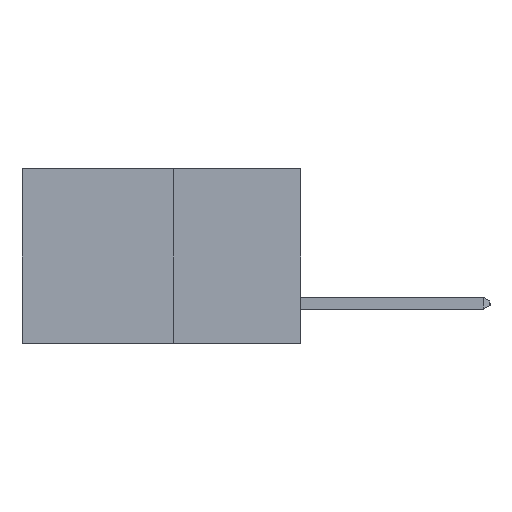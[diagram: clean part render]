
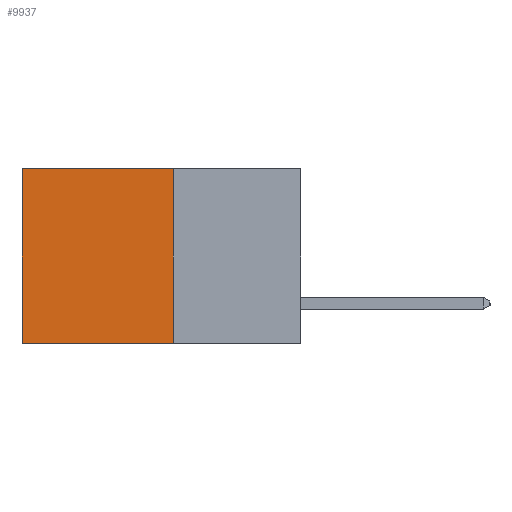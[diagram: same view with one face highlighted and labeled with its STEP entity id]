
A CAD part, left-side view. The second image highlights one B-rep face of the part: STEP entity #9937.
In plain terms, the highlighted planar face has unit normal (-1, 0, 0).
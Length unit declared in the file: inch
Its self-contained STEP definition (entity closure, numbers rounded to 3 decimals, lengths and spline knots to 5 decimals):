
#439 = EDGE_CURVE ( 'NONE', #6047, #4865, #7994, .T. ) ;
#1442 = FACE_OUTER_BOUND ( 'NONE', #7713, .T. ) ;
#1578 = LINE ( 'NONE', #4996, #12822 ) ;
#1787 = DIRECTION ( 'NONE',  ( 0., 1., 0. ) ) ;
#1858 = VECTOR ( 'NONE', #1787, 39.37008 ) ;
#2260 = CARTESIAN_POINT ( 'NONE',  ( 0.277, 0.59, 0. ) ) ;
#2309 = CARTESIAN_POINT ( 'NONE',  ( 0.277, 0.59, -0.37 ) ) ;
#2330 = EDGE_CURVE ( 'NONE', #6047, #13140, #10351, .T. ) ;
#2513 = CARTESIAN_POINT ( 'NONE',  ( 0.277, 0.27, -0.37 ) ) ;
#2877 = ORIENTED_EDGE ( 'NONE', *, *, #8731, .T. ) ;
#3456 = DIRECTION ( 'NONE',  ( 0., 0., -1. ) ) ;
#3607 = DIRECTION ( 'NONE',  ( 0., 0., -1. ) ) ;
#4017 = CARTESIAN_POINT ( 'NONE',  ( 0.277, 0.27, -0.37 ) ) ;
#4865 = VERTEX_POINT ( 'NONE', #2260 ) ;
#4996 = CARTESIAN_POINT ( 'NONE',  ( 0.277, 0.27, -0.37 ) ) ;
#5775 = CARTESIAN_POINT ( 'NONE',  ( 0.277, 0.27, 0. ) ) ;
#6047 = VERTEX_POINT ( 'NONE', #6711 ) ;
#6207 = ORIENTED_EDGE ( 'NONE', *, *, #2330, .F. ) ;
#6711 = CARTESIAN_POINT ( 'NONE',  ( 0.277, 0.27, 0. ) ) ;
#7179 = DIRECTION ( 'NONE',  ( 0., 1., 0. ) ) ;
#7713 = EDGE_LOOP ( 'NONE', ( #2877, #8982, #6207, #10293 ) ) ;
#7994 = LINE ( 'NONE', #5775, #1858 ) ;
#8449 = VECTOR ( 'NONE', #3456, 39.37008 ) ;
#8731 = EDGE_CURVE ( 'NONE', #4865, #13136, #11397, .T. ) ;
#8982 = ORIENTED_EDGE ( 'NONE', *, *, #11948, .F. ) ;
#9730 = AXIS2_PLACEMENT_3D ( 'NONE', #2513, #10194, #3607 ) ;
#9932 = CARTESIAN_POINT ( 'NONE',  ( 0.277, 0.27, -0.37 ) ) ;
#9937 = ADVANCED_FACE ( 'NONE', ( #1442 ), #11249, .F. ) ;
#10194 = DIRECTION ( 'NONE',  ( 1., 0., 0. ) ) ;
#10293 = ORIENTED_EDGE ( 'NONE', *, *, #439, .T. ) ;
#10351 = LINE ( 'NONE', #9932, #12879 ) ;
#11249 = PLANE ( 'NONE',  #9730 ) ;
#11397 = LINE ( 'NONE', #2309, #8449 ) ;
#11687 = CARTESIAN_POINT ( 'NONE',  ( 0.277, 0.59, -0.37 ) ) ;
#11948 = EDGE_CURVE ( 'NONE', #13140, #13136, #1578, .T. ) ;
#12271 = DIRECTION ( 'NONE',  ( 0., 0., -1. ) ) ;
#12822 = VECTOR ( 'NONE', #7179, 39.37008 ) ;
#12879 = VECTOR ( 'NONE', #12271, 39.37008 ) ;
#13136 = VERTEX_POINT ( 'NONE', #11687 ) ;
#13140 = VERTEX_POINT ( 'NONE', #4017 ) ;
